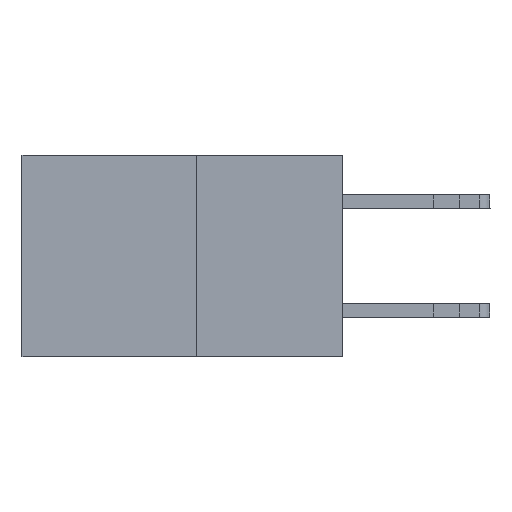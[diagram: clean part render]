
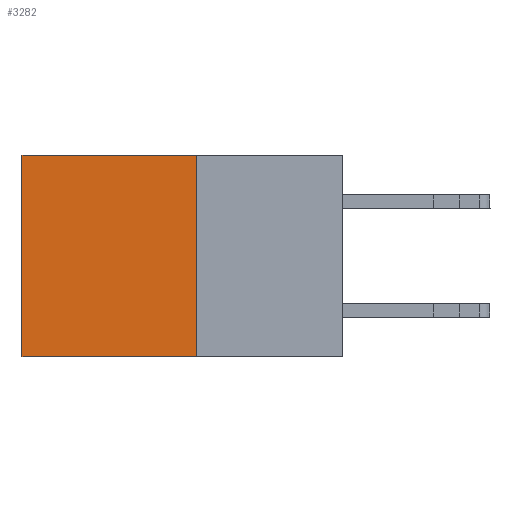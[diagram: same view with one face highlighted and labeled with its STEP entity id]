
A CAD part, left-side view. The second image highlights one B-rep face of the part: STEP entity #3282.
In plain terms, the highlighted planar face has unit normal (-1, 0, 0).
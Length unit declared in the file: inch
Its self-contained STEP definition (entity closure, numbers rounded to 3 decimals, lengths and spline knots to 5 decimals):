
#282 = LINE ( 'NONE', #1392, #3509 ) ;
#360 = VECTOR ( 'NONE', #7582, 39.37008 ) ;
#797 = DIRECTION ( 'NONE',  ( 0., 1., 0. ) ) ;
#1317 = DIRECTION ( 'NONE',  ( 1., 0., 0. ) ) ;
#1392 = CARTESIAN_POINT ( 'NONE',  ( 0.277, 0.27, -0.37 ) ) ;
#1502 = EDGE_CURVE ( 'NONE', #3704, #1994, #6427, .T. ) ;
#1588 = AXIS2_PLACEMENT_3D ( 'NONE', #11753, #1317, #8742 ) ;
#1806 = CARTESIAN_POINT ( 'NONE',  ( 0.277, 0.27, -0.37 ) ) ;
#1878 = ORIENTED_EDGE ( 'NONE', *, *, #4323, .T. ) ;
#1994 = VERTEX_POINT ( 'NONE', #1806 ) ;
#2102 = VERTEX_POINT ( 'NONE', #10529 ) ;
#2798 = LINE ( 'NONE', #13312, #7980 ) ;
#3282 = ADVANCED_FACE ( 'NONE', ( #3544 ), #9718, .F. ) ;
#3509 = VECTOR ( 'NONE', #3763, 39.37008 ) ;
#3544 = FACE_OUTER_BOUND ( 'NONE', #11209, .T. ) ;
#3704 = VERTEX_POINT ( 'NONE', #8511 ) ;
#3763 = DIRECTION ( 'NONE',  ( 0., 1., 0. ) ) ;
#4323 = EDGE_CURVE ( 'NONE', #3704, #5574, #2798, .T. ) ;
#4547 = ORIENTED_EDGE ( 'NONE', *, *, #12283, .T. ) ;
#4770 = EDGE_CURVE ( 'NONE', #1994, #2102, #282, .T. ) ;
#5515 = CARTESIAN_POINT ( 'NONE',  ( 0.277, 0.59, -0.37 ) ) ;
#5574 = VERTEX_POINT ( 'NONE', #10177 ) ;
#5805 = VECTOR ( 'NONE', #10847, 39.37008 ) ;
#5946 = ORIENTED_EDGE ( 'NONE', *, *, #1502, .F. ) ;
#6427 = LINE ( 'NONE', #11251, #5805 ) ;
#7582 = DIRECTION ( 'NONE',  ( 0., 0., -1. ) ) ;
#7980 = VECTOR ( 'NONE', #797, 39.37008 ) ;
#8511 = CARTESIAN_POINT ( 'NONE',  ( 0.277, 0.27, 0. ) ) ;
#8742 = DIRECTION ( 'NONE',  ( 0., 0., -1. ) ) ;
#8973 = LINE ( 'NONE', #5515, #360 ) ;
#9124 = ORIENTED_EDGE ( 'NONE', *, *, #4770, .F. ) ;
#9718 = PLANE ( 'NONE',  #1588 ) ;
#10177 = CARTESIAN_POINT ( 'NONE',  ( 0.277, 0.59, 0. ) ) ;
#10529 = CARTESIAN_POINT ( 'NONE',  ( 0.277, 0.59, -0.37 ) ) ;
#10847 = DIRECTION ( 'NONE',  ( 0., 0., -1. ) ) ;
#11209 = EDGE_LOOP ( 'NONE', ( #4547, #9124, #5946, #1878 ) ) ;
#11251 = CARTESIAN_POINT ( 'NONE',  ( 0.277, 0.27, -0.37 ) ) ;
#11753 = CARTESIAN_POINT ( 'NONE',  ( 0.277, 0.27, -0.37 ) ) ;
#12283 = EDGE_CURVE ( 'NONE', #5574, #2102, #8973, .T. ) ;
#13312 = CARTESIAN_POINT ( 'NONE',  ( 0.277, 0.27, 0. ) ) ;
